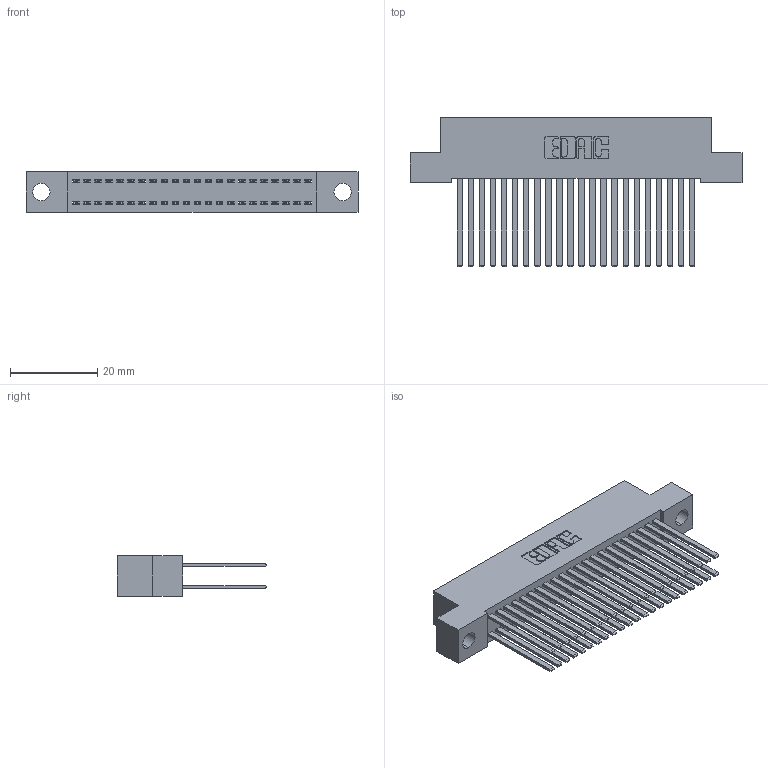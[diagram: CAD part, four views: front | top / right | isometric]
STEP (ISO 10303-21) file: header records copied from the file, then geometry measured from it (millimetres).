
FILE_DESCRIPTION (( 'STEP AP203' ), '1' );
FILE_NAME ('392-044-544-204.STEP', '2018-08-16T15:26:19', ( '' ), ( '' ), 'SwSTEP 2.0', 'SolidWorks 2016', '' );
FILE_SCHEMA (( 'CONFIG_CONTROL_DESIGN' ));
Length unit declared in the file: inch
Products named in the file (3): 342 Part_.156 TH; 345-292-001_345-293-144; 392-044-544-204
Assembly tree (45 placements, depth 2):
  392-044-544-204
    342 Part_.156 TH
    345-292-001_345-293-144  x44
Bounding box: 76.2 x 34.3 x 9.4 mm (x, y, z)
Volume: 7281.7 mm3; surface area: 12892.2 mm2
Topology: 45 solids, 45 shells, 2134 faces, 6327 edges, 4158 vertices
Faces by surface type: plane 1474, cylinder 660
Entity records: 16427 total; most frequent: CARTESIAN_POINT 2742, ORIENTED_EDGE 2678, DIRECTION 2375, EDGE_CURVE 1339, VECTOR 1215, LINE 1215, VERTEX_POINT 890, AXIS2_PLACEMENT_3D 580
